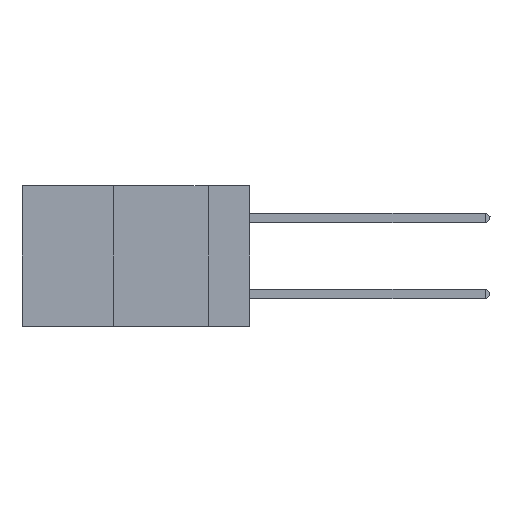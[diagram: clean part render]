
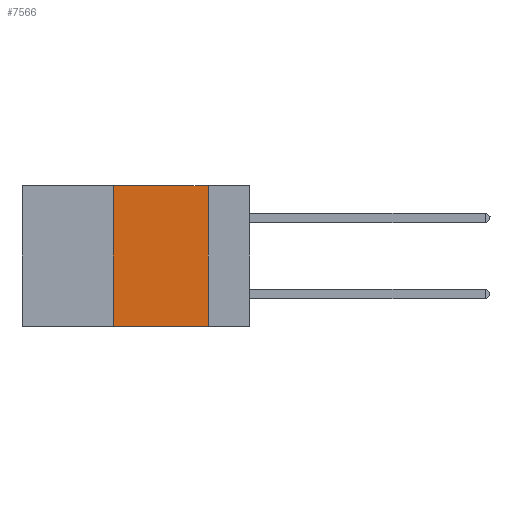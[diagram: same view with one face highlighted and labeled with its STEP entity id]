
A CAD part, left-side view. The second image highlights one B-rep face of the part: STEP entity #7566.
In plain terms, the highlighted planar face has unit normal (-1, 0, 0).
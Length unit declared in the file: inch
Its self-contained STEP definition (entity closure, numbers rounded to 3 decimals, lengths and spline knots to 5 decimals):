
#330 = CARTESIAN_POINT ( 'NONE',  ( 0., 0.6, 0. ) ) ;
#2708 = ORIENTED_EDGE ( 'NONE', *, *, #27818, .F. ) ;
#3128 = ORIENTED_EDGE ( 'NONE', *, *, #7528, .F. ) ;
#3146 = DIRECTION ( 'NONE',  ( 1., 0., 0. ) ) ;
#3545 = VERTEX_POINT ( 'NONE', #5199 ) ;
#3766 = FACE_OUTER_BOUND ( 'NONE', #4536, .T. ) ;
#4536 = EDGE_LOOP ( 'NONE', ( #2708, #3128, #7852, #16350 ) ) ;
#4764 = CARTESIAN_POINT ( 'NONE',  ( 0., 0.11, -0.37 ) ) ;
#5199 = CARTESIAN_POINT ( 'NONE',  ( 0., 0.36, -0.37 ) ) ;
#5730 = VERTEX_POINT ( 'NONE', #31903 ) ;
#6106 = CARTESIAN_POINT ( 'NONE',  ( 0., 0.36, 0. ) ) ;
#7407 = LINE ( 'NONE', #8329, #23889 ) ;
#7489 = AXIS2_PLACEMENT_3D ( 'NONE', #330, #3146, #27890 ) ;
#7528 = EDGE_CURVE ( 'NONE', #35132, #5730, #10182, .T. ) ;
#7566 = ADVANCED_FACE ( 'NONE', ( #3766 ), #25128, .F. ) ;
#7852 = ORIENTED_EDGE ( 'NONE', *, *, #26328, .F. ) ;
#8329 = CARTESIAN_POINT ( 'NONE',  ( 0., 0.11, 0. ) ) ;
#10182 = LINE ( 'NONE', #19572, #26651 ) ;
#10923 = LINE ( 'NONE', #23612, #17449 ) ;
#13022 = EDGE_CURVE ( 'NONE', #3545, #21716, #21270, .T. ) ;
#16350 = ORIENTED_EDGE ( 'NONE', *, *, #13022, .T. ) ;
#17449 = VECTOR ( 'NONE', #34787, 39.37008 ) ;
#18165 = DIRECTION ( 'NONE',  ( 0., -1., 0. ) ) ;
#19572 = CARTESIAN_POINT ( 'NONE',  ( 0., 0.6, 0. ) ) ;
#21270 = LINE ( 'NONE', #34066, #32069 ) ;
#21716 = VERTEX_POINT ( 'NONE', #4764 ) ;
#23612 = CARTESIAN_POINT ( 'NONE',  ( 0., 0.36, 0. ) ) ;
#23889 = VECTOR ( 'NONE', #25621, 39.37008 ) ;
#25128 = PLANE ( 'NONE',  #7489 ) ;
#25621 = DIRECTION ( 'NONE',  ( 0., 0., -1. ) ) ;
#26328 = EDGE_CURVE ( 'NONE', #3545, #35132, #10923, .T. ) ;
#26651 = VECTOR ( 'NONE', #27771, 39.37008 ) ;
#27771 = DIRECTION ( 'NONE',  ( 0., -1., 0. ) ) ;
#27818 = EDGE_CURVE ( 'NONE', #5730, #21716, #7407, .T. ) ;
#27890 = DIRECTION ( 'NONE',  ( 0., 0., -1. ) ) ;
#31903 = CARTESIAN_POINT ( 'NONE',  ( 0., 0.11, 0. ) ) ;
#32069 = VECTOR ( 'NONE', #18165, 39.37008 ) ;
#34066 = CARTESIAN_POINT ( 'NONE',  ( 0., 0.6, -0.37 ) ) ;
#34787 = DIRECTION ( 'NONE',  ( 0., 0., 1. ) ) ;
#35132 = VERTEX_POINT ( 'NONE', #6106 ) ;
